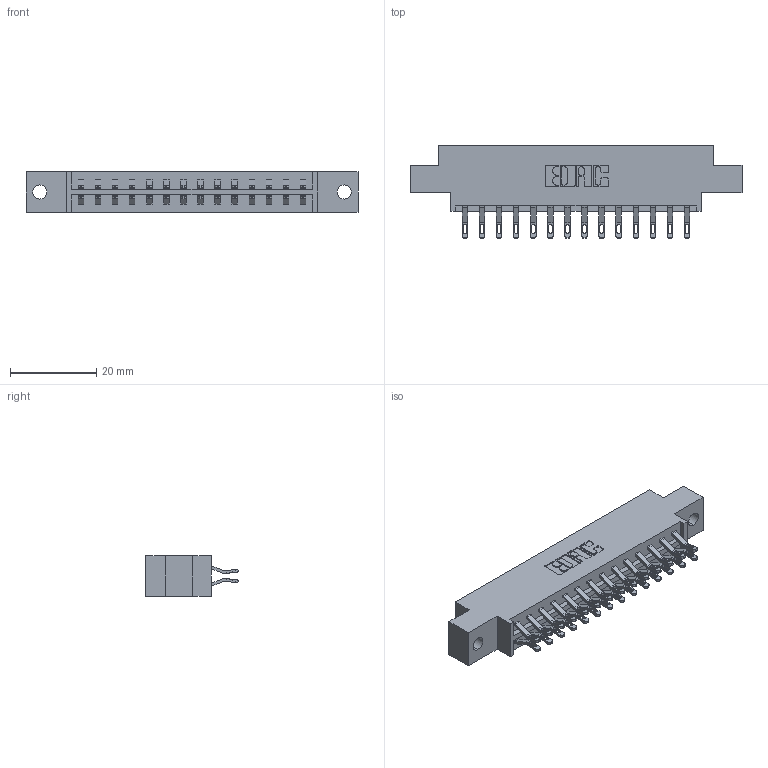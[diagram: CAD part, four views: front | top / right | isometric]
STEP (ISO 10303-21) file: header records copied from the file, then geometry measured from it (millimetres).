
FILE_DESCRIPTION (( 'STEP AP203' ), '1' );
FILE_NAME ('333-028-555-802.STEP', '2018-08-02T15:37:57', ( '' ), ( '' ), 'SwSTEP 2.0', 'SolidWorks 2016', '' );
FILE_SCHEMA (( 'CONFIG_CONTROL_DESIGN' ));
Length unit declared in the file: inch
Products named in the file (3): 333 Part_Offset - .128 Dia; 345-292-001_555 Tail; 333-028-555-802
Assembly tree (29 placements, depth 2):
  333-028-555-802
    333 Part_Offset - .128 Dia
    345-292-001_555 Tail  x28
Bounding box: 77.01 x 21.47 x 9.4 mm (x, y, z)
Volume: 7417.5 mm3; surface area: 8719.6 mm2
Topology: 29 solids, 29 shells, 1742 faces, 5447 edges, 3630 vertices
Faces by surface type: plane 1026, cylinder 716
Entity records: 13089 total; most frequent: CARTESIAN_POINT 2240, ORIENTED_EDGE 2146, DIRECTION 1933, EDGE_CURVE 1073, LINE 925, VECTOR 925, VERTEX_POINT 714, AXIS2_PLACEMENT_3D 504
